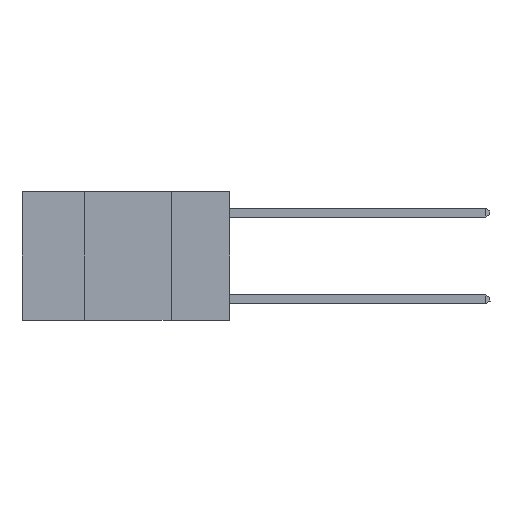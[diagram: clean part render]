
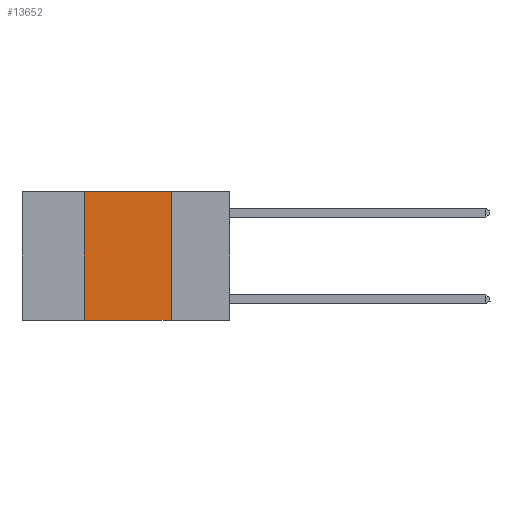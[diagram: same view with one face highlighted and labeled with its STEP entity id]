
A CAD part, left-side view. The second image highlights one B-rep face of the part: STEP entity #13652.
In plain terms, the highlighted planar face has unit normal (-1, 0, 0).
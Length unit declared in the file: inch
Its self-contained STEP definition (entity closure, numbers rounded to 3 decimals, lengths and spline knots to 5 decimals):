
#462 = LINE ( 'NONE', #14448, #19842 ) ;
#741 = CARTESIAN_POINT ( 'NONE',  ( 0., 0.6, -0.37 ) ) ;
#871 = CARTESIAN_POINT ( 'NONE',  ( 0., 0.6, 0. ) ) ;
#933 = VECTOR ( 'NONE', #19866, 39.37008 ) ;
#2154 = ORIENTED_EDGE ( 'NONE', *, *, #13592, .T. ) ;
#2362 = DIRECTION ( 'NONE',  ( 0., -1., 0. ) ) ;
#2495 = DIRECTION ( 'NONE',  ( 0., 0., -1. ) ) ;
#2682 = VERTEX_POINT ( 'NONE', #9847 ) ;
#3381 = EDGE_CURVE ( 'NONE', #2682, #19340, #10261, .T. ) ;
#5387 = VECTOR ( 'NONE', #13546, 39.37008 ) ;
#5766 = AXIS2_PLACEMENT_3D ( 'NONE', #871, #11873, #2495 ) ;
#6319 = ORIENTED_EDGE ( 'NONE', *, *, #14633, .F. ) ;
#6639 = DIRECTION ( 'NONE',  ( 0., 0., 1. ) ) ;
#6803 = VERTEX_POINT ( 'NONE', #15999 ) ;
#6865 = EDGE_LOOP ( 'NONE', ( #12216, #19551, #6319, #2154 ) ) ;
#8879 = FACE_OUTER_BOUND ( 'NONE', #6865, .T. ) ;
#9847 = CARTESIAN_POINT ( 'NONE',  ( 0., 0.42, 0. ) ) ;
#10261 = LINE ( 'NONE', #12990, #933 ) ;
#10328 = LINE ( 'NONE', #741, #15013 ) ;
#11873 = DIRECTION ( 'NONE',  ( 1., 0., 0. ) ) ;
#11955 = CARTESIAN_POINT ( 'NONE',  ( 0., 0.17, 0. ) ) ;
#12216 = ORIENTED_EDGE ( 'NONE', *, *, #17749, .F. ) ;
#12990 = CARTESIAN_POINT ( 'NONE',  ( 0., 0.6, 0. ) ) ;
#13546 = DIRECTION ( 'NONE',  ( 0., 0., -1. ) ) ;
#13592 = EDGE_CURVE ( 'NONE', #6803, #17277, #10328, .T. ) ;
#13652 = ADVANCED_FACE ( 'NONE', ( #8879 ), #19655, .F. ) ;
#14448 = CARTESIAN_POINT ( 'NONE',  ( 0., 0.42, 0. ) ) ;
#14633 = EDGE_CURVE ( 'NONE', #6803, #2682, #462, .T. ) ;
#15013 = VECTOR ( 'NONE', #2362, 39.37008 ) ;
#15535 = CARTESIAN_POINT ( 'NONE',  ( 0., 0.17, -0.37 ) ) ;
#15999 = CARTESIAN_POINT ( 'NONE',  ( 0., 0.42, -0.37 ) ) ;
#17277 = VERTEX_POINT ( 'NONE', #15535 ) ;
#17749 = EDGE_CURVE ( 'NONE', #19340, #17277, #17861, .T. ) ;
#17861 = LINE ( 'NONE', #11955, #5387 ) ;
#18949 = CARTESIAN_POINT ( 'NONE',  ( 0., 0.17, 0. ) ) ;
#19340 = VERTEX_POINT ( 'NONE', #18949 ) ;
#19551 = ORIENTED_EDGE ( 'NONE', *, *, #3381, .F. ) ;
#19655 = PLANE ( 'NONE',  #5766 ) ;
#19842 = VECTOR ( 'NONE', #6639, 39.37008 ) ;
#19866 = DIRECTION ( 'NONE',  ( 0., -1., 0. ) ) ;
